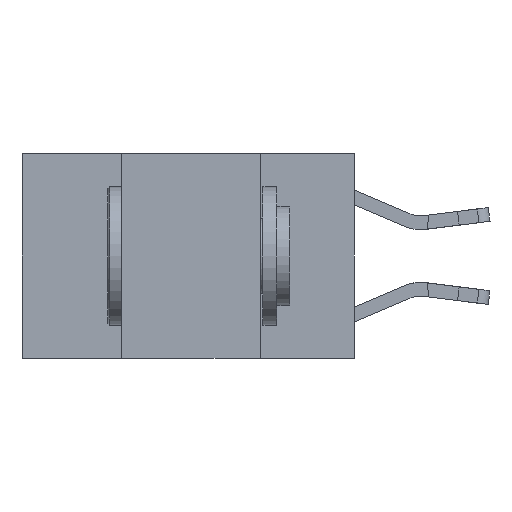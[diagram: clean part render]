
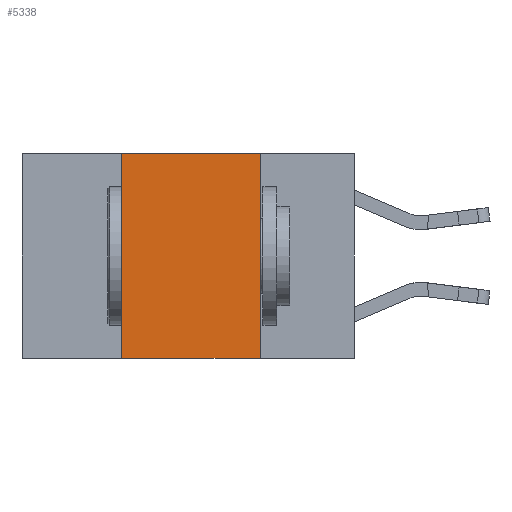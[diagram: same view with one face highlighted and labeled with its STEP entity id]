
A CAD part, left-side view. The second image highlights one B-rep face of the part: STEP entity #5338.
In plain terms, the highlighted planar face has unit normal (-1, 0, 0).
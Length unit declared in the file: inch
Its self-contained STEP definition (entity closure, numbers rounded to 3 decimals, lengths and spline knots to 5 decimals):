
#194 = CARTESIAN_POINT ( 'NONE',  ( 0., 0.17, 0. ) ) ;
#248 = EDGE_CURVE ( 'NONE', #11606, #4623, #15053, .T. ) ;
#792 = LINE ( 'NONE', #5971, #12833 ) ;
#910 = CARTESIAN_POINT ( 'NONE',  ( 0., 0.17, 0. ) ) ;
#1490 = FACE_OUTER_BOUND ( 'NONE', #3480, .T. ) ;
#1525 = DIRECTION ( 'NONE',  ( 0., -1., 0. ) ) ;
#2055 = ORIENTED_EDGE ( 'NONE', *, *, #8506, .F. ) ;
#2659 = CARTESIAN_POINT ( 'NONE',  ( 0., 0.6, -0.37 ) ) ;
#3044 = VERTEX_POINT ( 'NONE', #3229 ) ;
#3229 = CARTESIAN_POINT ( 'NONE',  ( 0., 0.42, 0. ) ) ;
#3480 = EDGE_LOOP ( 'NONE', ( #7941, #2055, #5170, #8298 ) ) ;
#4101 = CARTESIAN_POINT ( 'NONE',  ( 0., 0.42, 0. ) ) ;
#4392 = CARTESIAN_POINT ( 'NONE',  ( 0., 0.17, -0.37 ) ) ;
#4470 = PLANE ( 'NONE',  #14921 ) ;
#4526 = DIRECTION ( 'NONE',  ( 1., 0., 0. ) ) ;
#4623 = VERTEX_POINT ( 'NONE', #4392 ) ;
#5170 = ORIENTED_EDGE ( 'NONE', *, *, #7566, .F. ) ;
#5338 = ADVANCED_FACE ( 'NONE', ( #1490 ), #4470, .F. ) ;
#5971 = CARTESIAN_POINT ( 'NONE',  ( 0., 0.6, 0. ) ) ;
#6325 = DIRECTION ( 'NONE',  ( 0., 0., -1. ) ) ;
#6788 = EDGE_CURVE ( 'NONE', #7357, #4623, #8767, .T. ) ;
#7357 = VERTEX_POINT ( 'NONE', #12965 ) ;
#7566 = EDGE_CURVE ( 'NONE', #7357, #3044, #10557, .T. ) ;
#7836 = VECTOR ( 'NONE', #14493, 39.37008 ) ;
#7941 = ORIENTED_EDGE ( 'NONE', *, *, #248, .F. ) ;
#8298 = ORIENTED_EDGE ( 'NONE', *, *, #6788, .T. ) ;
#8391 = VECTOR ( 'NONE', #1525, 39.37008 ) ;
#8506 = EDGE_CURVE ( 'NONE', #3044, #11606, #792, .T. ) ;
#8767 = LINE ( 'NONE', #2659, #8391 ) ;
#8979 = VECTOR ( 'NONE', #6325, 39.37008 ) ;
#9498 = DIRECTION ( 'NONE',  ( 0., -1., 0. ) ) ;
#10557 = LINE ( 'NONE', #4101, #7836 ) ;
#11474 = CARTESIAN_POINT ( 'NONE',  ( 0., 0.6, 0. ) ) ;
#11606 = VERTEX_POINT ( 'NONE', #910 ) ;
#12619 = DIRECTION ( 'NONE',  ( 0., 0., -1. ) ) ;
#12833 = VECTOR ( 'NONE', #9498, 39.37008 ) ;
#12965 = CARTESIAN_POINT ( 'NONE',  ( 0., 0.42, -0.37 ) ) ;
#14493 = DIRECTION ( 'NONE',  ( 0., 0., 1. ) ) ;
#14921 = AXIS2_PLACEMENT_3D ( 'NONE', #11474, #4526, #12619 ) ;
#15053 = LINE ( 'NONE', #194, #8979 ) ;
